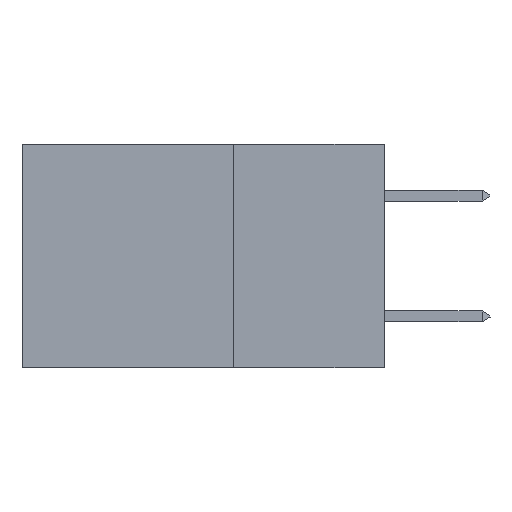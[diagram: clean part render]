
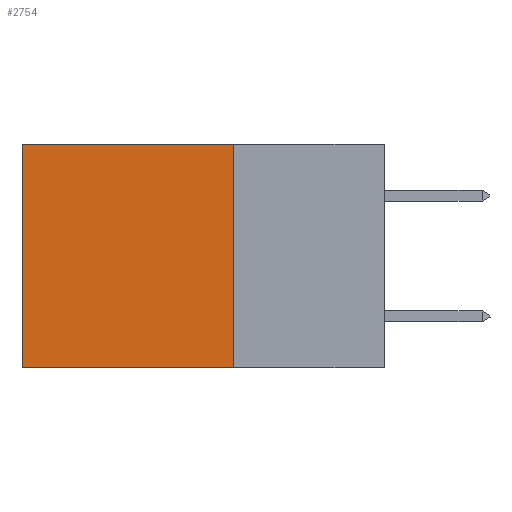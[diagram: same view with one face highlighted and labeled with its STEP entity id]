
A CAD part, left-side view. The second image highlights one B-rep face of the part: STEP entity #2754.
In plain terms, the highlighted planar face has unit normal (-1, 0, 0).
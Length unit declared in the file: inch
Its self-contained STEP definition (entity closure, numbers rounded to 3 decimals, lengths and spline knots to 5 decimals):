
#401 = VECTOR ( 'NONE', #17765, 39.37008 ) ;
#1303 = CARTESIAN_POINT ( 'NONE',  ( 0.2875, 0.6, -0.37 ) ) ;
#1417 = VECTOR ( 'NONE', #2807, 39.37008 ) ;
#2754 = ADVANCED_FACE ( 'NONE', ( #26040 ), #27825, .F. ) ;
#2807 = DIRECTION ( 'NONE',  ( 0., 0., -1. ) ) ;
#2850 = CARTESIAN_POINT ( 'NONE',  ( 0.2875, 0.25, 0. ) ) ;
#3241 = VERTEX_POINT ( 'NONE', #6326 ) ;
#3803 = DIRECTION ( 'NONE',  ( 0., 1., 0. ) ) ;
#6140 = CARTESIAN_POINT ( 'NONE',  ( 0.2875, 0.25, 0. ) ) ;
#6326 = CARTESIAN_POINT ( 'NONE',  ( 0.2875, 0.6, 0. ) ) ;
#7894 = CARTESIAN_POINT ( 'NONE',  ( 0.2875, 0.25, 0. ) ) ;
#8077 = ORIENTED_EDGE ( 'NONE', *, *, #24970, .T. ) ;
#8135 = LINE ( 'NONE', #25552, #1417 ) ;
#9200 = VERTEX_POINT ( 'NONE', #2850 ) ;
#10169 = VECTOR ( 'NONE', #23341, 39.37008 ) ;
#10924 = EDGE_LOOP ( 'NONE', ( #8077, #16864, #20700, #17391 ) ) ;
#12610 = DIRECTION ( 'NONE',  ( 1., 0., 0. ) ) ;
#12863 = EDGE_CURVE ( 'NONE', #17869, #21787, #31779, .T. ) ;
#13066 = CARTESIAN_POINT ( 'NONE',  ( 0.2875, 0.25, -0.37 ) ) ;
#13307 = LINE ( 'NONE', #15748, #10169 ) ;
#13361 = AXIS2_PLACEMENT_3D ( 'NONE', #7894, #12610, #27405 ) ;
#15748 = CARTESIAN_POINT ( 'NONE',  ( 0.2875, 0.25, 0. ) ) ;
#16864 = ORIENTED_EDGE ( 'NONE', *, *, #12863, .F. ) ;
#16872 = CARTESIAN_POINT ( 'NONE',  ( 0.2875, 0.25, -0.37 ) ) ;
#17391 = ORIENTED_EDGE ( 'NONE', *, *, #18898, .T. ) ;
#17733 = EDGE_CURVE ( 'NONE', #9200, #17869, #13307, .T. ) ;
#17765 = DIRECTION ( 'NONE',  ( 0., 1., 0. ) ) ;
#17869 = VERTEX_POINT ( 'NONE', #16872 ) ;
#18898 = EDGE_CURVE ( 'NONE', #9200, #3241, #27721, .T. ) ;
#20700 = ORIENTED_EDGE ( 'NONE', *, *, #17733, .F. ) ;
#21787 = VERTEX_POINT ( 'NONE', #1303 ) ;
#23341 = DIRECTION ( 'NONE',  ( 0., 0., -1. ) ) ;
#24970 = EDGE_CURVE ( 'NONE', #3241, #21787, #8135, .T. ) ;
#25552 = CARTESIAN_POINT ( 'NONE',  ( 0.2875, 0.6, 0. ) ) ;
#26040 = FACE_OUTER_BOUND ( 'NONE', #10924, .T. ) ;
#27405 = DIRECTION ( 'NONE',  ( 0., 0., -1. ) ) ;
#27721 = LINE ( 'NONE', #6140, #31991 ) ;
#27825 = PLANE ( 'NONE',  #13361 ) ;
#31779 = LINE ( 'NONE', #13066, #401 ) ;
#31991 = VECTOR ( 'NONE', #3803, 39.37008 ) ;
